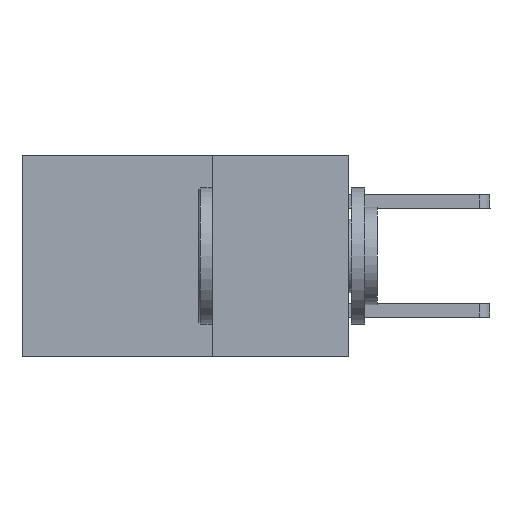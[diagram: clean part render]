
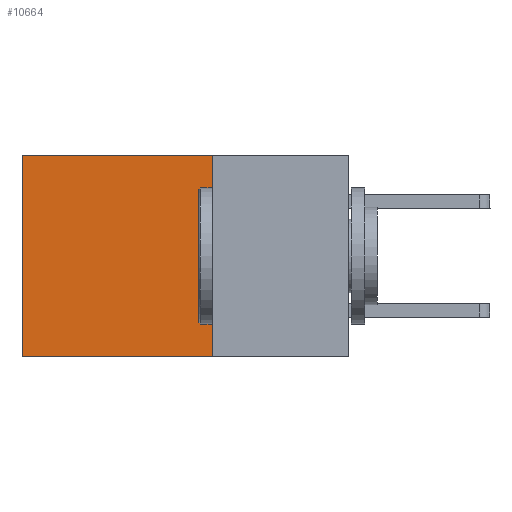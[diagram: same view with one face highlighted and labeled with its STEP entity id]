
A CAD part, left-side view. The second image highlights one B-rep face of the part: STEP entity #10664.
In plain terms, the highlighted planar face has unit normal (-1, 0, 0).
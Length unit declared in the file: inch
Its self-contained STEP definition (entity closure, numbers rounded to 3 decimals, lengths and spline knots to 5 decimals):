
#69 = CARTESIAN_POINT ( 'NONE',  ( 0.298, 0.25, -0.37 ) ) ;
#369 = EDGE_CURVE ( 'NONE', #8347, #9274, #10222, .T. ) ;
#618 = VERTEX_POINT ( 'NONE', #3823 ) ;
#1168 = CARTESIAN_POINT ( 'NONE',  ( 0.298, 0.25, -0.37 ) ) ;
#1758 = VECTOR ( 'NONE', #1947, 39.37008 ) ;
#1821 = CARTESIAN_POINT ( 'NONE',  ( 0.298, 0.25, 0. ) ) ;
#1947 = DIRECTION ( 'NONE',  ( 0., 0., -1. ) ) ;
#1997 = EDGE_CURVE ( 'NONE', #9274, #618, #6283, .T. ) ;
#2627 = CARTESIAN_POINT ( 'NONE',  ( 0.298, 0.6, 0. ) ) ;
#3147 = CARTESIAN_POINT ( 'NONE',  ( 0.298, 0.25, 0. ) ) ;
#3490 = EDGE_CURVE ( 'NONE', #8347, #3533, #3887, .T. ) ;
#3533 = VERTEX_POINT ( 'NONE', #1168 ) ;
#3823 = CARTESIAN_POINT ( 'NONE',  ( 0.298, 0.6, -0.37 ) ) ;
#3887 = LINE ( 'NONE', #3147, #10705 ) ;
#4702 = CARTESIAN_POINT ( 'NONE',  ( 0.298, 0.25, 0. ) ) ;
#4956 = CARTESIAN_POINT ( 'NONE',  ( 0.298, 0.25, 0. ) ) ;
#5304 = CARTESIAN_POINT ( 'NONE',  ( 0.298, 0.6, 0. ) ) ;
#5389 = VECTOR ( 'NONE', #10981, 39.37008 ) ;
#5607 = EDGE_CURVE ( 'NONE', #3533, #618, #7858, .T. ) ;
#5932 = VECTOR ( 'NONE', #9641, 39.37008 ) ;
#6047 = AXIS2_PLACEMENT_3D ( 'NONE', #4702, #9765, #9818 ) ;
#6283 = LINE ( 'NONE', #5304, #1758 ) ;
#6565 = DIRECTION ( 'NONE',  ( 0., 0., -1. ) ) ;
#7261 = ORIENTED_EDGE ( 'NONE', *, *, #1997, .T. ) ;
#7858 = LINE ( 'NONE', #69, #5932 ) ;
#8076 = PLANE ( 'NONE',  #6047 ) ;
#8347 = VERTEX_POINT ( 'NONE', #1821 ) ;
#9274 = VERTEX_POINT ( 'NONE', #2627 ) ;
#9516 = ORIENTED_EDGE ( 'NONE', *, *, #3490, .F. ) ;
#9641 = DIRECTION ( 'NONE',  ( 0., 1., 0. ) ) ;
#9765 = DIRECTION ( 'NONE',  ( 1., 0., 0. ) ) ;
#9818 = DIRECTION ( 'NONE',  ( 0., 0., -1. ) ) ;
#10099 = ORIENTED_EDGE ( 'NONE', *, *, #369, .T. ) ;
#10222 = LINE ( 'NONE', #4956, #5389 ) ;
#10664 = ADVANCED_FACE ( 'NONE', ( #10848 ), #8076, .F. ) ;
#10705 = VECTOR ( 'NONE', #6565, 39.37008 ) ;
#10787 = ORIENTED_EDGE ( 'NONE', *, *, #5607, .F. ) ;
#10847 = EDGE_LOOP ( 'NONE', ( #7261, #10787, #9516, #10099 ) ) ;
#10848 = FACE_OUTER_BOUND ( 'NONE', #10847, .T. ) ;
#10981 = DIRECTION ( 'NONE',  ( 0., 1., 0. ) ) ;
